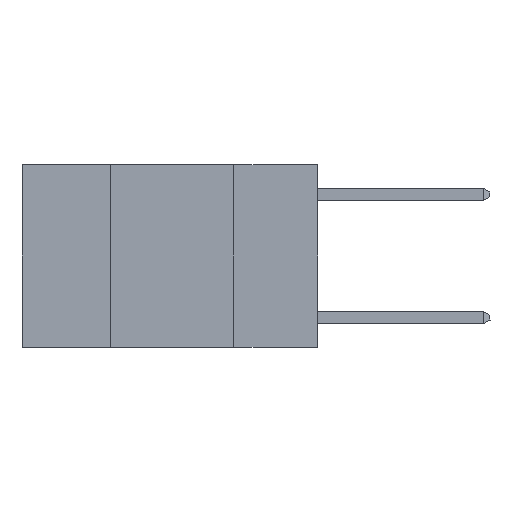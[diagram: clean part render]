
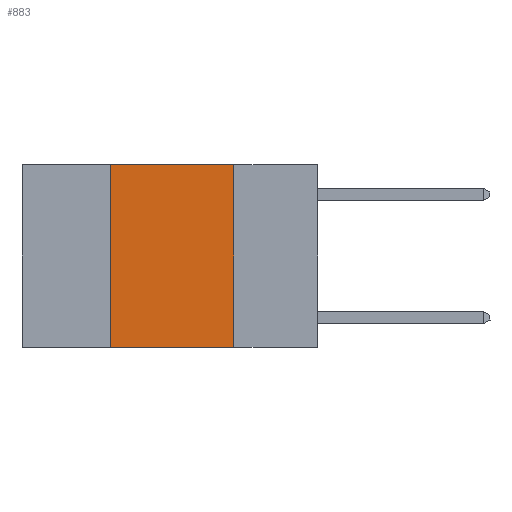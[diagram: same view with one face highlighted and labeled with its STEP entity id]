
A CAD part, left-side view. The second image highlights one B-rep face of the part: STEP entity #883.
In plain terms, the highlighted planar face has unit normal (-1, 0, 0).
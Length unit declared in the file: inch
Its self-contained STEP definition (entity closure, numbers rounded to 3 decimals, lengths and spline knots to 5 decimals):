
#123 = DIRECTION ( 'NONE',  ( 0., -1., 0. ) ) ;
#408 = VECTOR ( 'NONE', #4927, 39.37008 ) ;
#486 = CARTESIAN_POINT ( 'NONE',  ( 0., 0.17, 0. ) ) ;
#883 = ADVANCED_FACE ( 'NONE', ( #9994 ), #9760, .F. ) ;
#1051 = CARTESIAN_POINT ( 'NONE',  ( 0., 0.17, -0.37 ) ) ;
#1646 = VERTEX_POINT ( 'NONE', #486 ) ;
#1796 = VERTEX_POINT ( 'NONE', #4440 ) ;
#2024 = ORIENTED_EDGE ( 'NONE', *, *, #7740, .F. ) ;
#3030 = ORIENTED_EDGE ( 'NONE', *, *, #6617, .F. ) ;
#3673 = CARTESIAN_POINT ( 'NONE',  ( 0., 0.42, 0. ) ) ;
#3683 = VECTOR ( 'NONE', #7171, 39.37008 ) ;
#4038 = ORIENTED_EDGE ( 'NONE', *, *, #10804, .F. ) ;
#4323 = DIRECTION ( 'NONE',  ( 1., 0., 0. ) ) ;
#4440 = CARTESIAN_POINT ( 'NONE',  ( 0., 0.42, -0.37 ) ) ;
#4539 = VECTOR ( 'NONE', #123, 39.37008 ) ;
#4927 = DIRECTION ( 'NONE',  ( 0., 0., -1. ) ) ;
#5055 = LINE ( 'NONE', #11103, #408 ) ;
#5378 = EDGE_LOOP ( 'NONE', ( #2024, #4038, #3030, #6590 ) ) ;
#5941 = CARTESIAN_POINT ( 'NONE',  ( 0., 0.6, -0.37 ) ) ;
#6000 = LINE ( 'NONE', #3673, #3683 ) ;
#6247 = VERTEX_POINT ( 'NONE', #7652 ) ;
#6549 = CARTESIAN_POINT ( 'NONE',  ( 0., 0.6, 0. ) ) ;
#6590 = ORIENTED_EDGE ( 'NONE', *, *, #10338, .T. ) ;
#6594 = LINE ( 'NONE', #5941, #8643 ) ;
#6617 = EDGE_CURVE ( 'NONE', #1796, #6247, #6000, .T. ) ;
#7171 = DIRECTION ( 'NONE',  ( 0., 0., 1. ) ) ;
#7652 = CARTESIAN_POINT ( 'NONE',  ( 0., 0.42, 0. ) ) ;
#7699 = DIRECTION ( 'NONE',  ( 0., -1., 0. ) ) ;
#7740 = EDGE_CURVE ( 'NONE', #1646, #8635, #5055, .T. ) ;
#8635 = VERTEX_POINT ( 'NONE', #1051 ) ;
#8643 = VECTOR ( 'NONE', #7699, 39.37008 ) ;
#9211 = LINE ( 'NONE', #6549, #4539 ) ;
#9248 = CARTESIAN_POINT ( 'NONE',  ( 0., 0.6, 0. ) ) ;
#9760 = PLANE ( 'NONE',  #10697 ) ;
#9994 = FACE_OUTER_BOUND ( 'NONE', #5378, .T. ) ;
#10338 = EDGE_CURVE ( 'NONE', #1796, #8635, #6594, .T. ) ;
#10697 = AXIS2_PLACEMENT_3D ( 'NONE', #9248, #4323, #11072 ) ;
#10804 = EDGE_CURVE ( 'NONE', #6247, #1646, #9211, .T. ) ;
#11072 = DIRECTION ( 'NONE',  ( 0., 0., -1. ) ) ;
#11103 = CARTESIAN_POINT ( 'NONE',  ( 0., 0.17, 0. ) ) ;
